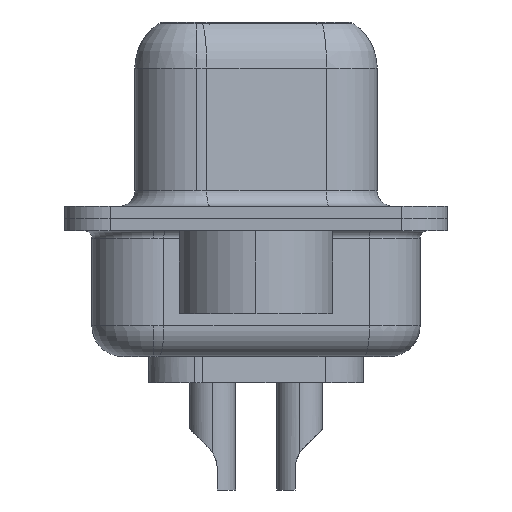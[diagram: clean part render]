
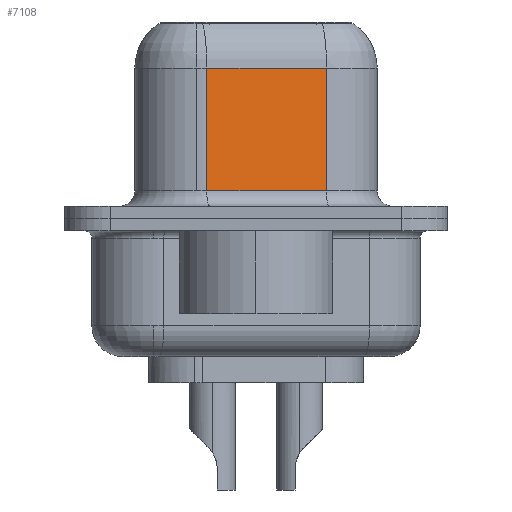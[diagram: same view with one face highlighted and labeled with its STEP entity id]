
A CAD part, left-side view. The second image highlights one B-rep face of the part: STEP entity #7108.
In plain terms, the highlighted planar face has unit normal (-0.985, -0.174, 0).
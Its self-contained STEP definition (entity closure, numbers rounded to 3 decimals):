
#61 = VERTEX_POINT ( 'NONE', #6378 ) ;
#829 = DIRECTION ( 'NONE',  ( -0.174, 0.985, 0. ) ) ;
#883 = CARTESIAN_POINT ( 'NONE',  ( 5.068, -2.297, 0.9 ) ) ;
#1876 = CARTESIAN_POINT ( 'NONE',  ( 5.068, -2.297, 4.9 ) ) ;
#2014 = FACE_OUTER_BOUND ( 'NONE', #6623, .T. ) ;
#2824 = AXIS2_PLACEMENT_3D ( 'NONE', #9404, #10431, #829 ) ;
#2851 = DIRECTION ( 'NONE',  ( 0., 0., -1. ) ) ;
#2863 = ORIENTED_EDGE ( 'NONE', *, *, #11549, .T. ) ;
#4027 = LINE ( 'NONE', #1876, #6606 ) ;
#5833 = CARTESIAN_POINT ( 'NONE',  ( 4.38, 1.603, 6.65 ) ) ;
#6364 = VERTEX_POINT ( 'NONE', #13546 ) ;
#6378 = CARTESIAN_POINT ( 'NONE',  ( 5.068, -2.297, 4.9 ) ) ;
#6478 = EDGE_CURVE ( 'NONE', #61, #12665, #4027, .T. ) ;
#6529 = DIRECTION ( 'NONE',  ( 0.174, -0.985, 0. ) ) ;
#6606 = VECTOR ( 'NONE', #15020, 1000. ) ;
#6623 = EDGE_LOOP ( 'NONE', ( #14055, #12480, #10906, #2863 ) ) ;
#6786 = VECTOR ( 'NONE', #13139, 1000. ) ;
#7108 = ADVANCED_FACE ( 'NONE', ( #2014 ), #11772, .F. ) ;
#7188 = LINE ( 'NONE', #5833, #6786 ) ;
#7711 = LINE ( 'NONE', #14824, #11047 ) ;
#8091 = EDGE_CURVE ( 'NONE', #12665, #6364, #7188, .T. ) ;
#8921 = CARTESIAN_POINT ( 'NONE',  ( 4.38, 1.603, 4.9 ) ) ;
#9404 = CARTESIAN_POINT ( 'NONE',  ( 5.068, -2.297, 6.65 ) ) ;
#10431 = DIRECTION ( 'NONE',  ( 0.985, 0.174, 0. ) ) ;
#10906 = ORIENTED_EDGE ( 'NONE', *, *, #8091, .T. ) ;
#11047 = VECTOR ( 'NONE', #6529, 1000. ) ;
#11549 = EDGE_CURVE ( 'NONE', #6364, #14528, #7711, .T. ) ;
#11772 = PLANE ( 'NONE',  #2824 ) ;
#12060 = EDGE_CURVE ( 'NONE', #61, #14528, #14963, .T. ) ;
#12087 = VECTOR ( 'NONE', #2851, 1000. ) ;
#12480 = ORIENTED_EDGE ( 'NONE', *, *, #6478, .T. ) ;
#12665 = VERTEX_POINT ( 'NONE', #8921 ) ;
#13139 = DIRECTION ( 'NONE',  ( 0., 0., -1. ) ) ;
#13546 = CARTESIAN_POINT ( 'NONE',  ( 4.38, 1.603, 0.9 ) ) ;
#13715 = CARTESIAN_POINT ( 'NONE',  ( 5.068, -2.297, 6.65 ) ) ;
#14055 = ORIENTED_EDGE ( 'NONE', *, *, #12060, .F. ) ;
#14528 = VERTEX_POINT ( 'NONE', #883 ) ;
#14824 = CARTESIAN_POINT ( 'NONE',  ( 5.068, -2.297, 0.9 ) ) ;
#14963 = LINE ( 'NONE', #13715, #12087 ) ;
#15020 = DIRECTION ( 'NONE',  ( -0.174, 0.985, 0. ) ) ;
